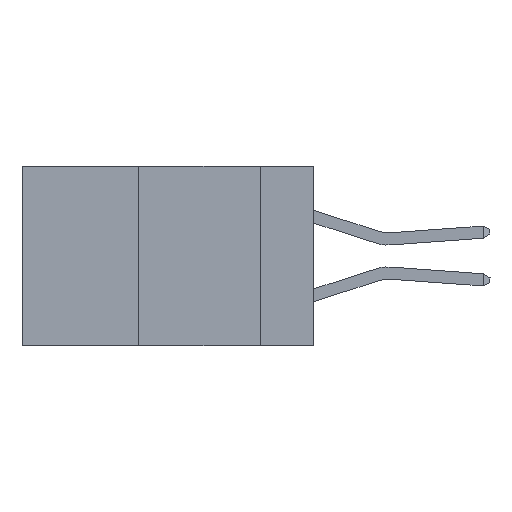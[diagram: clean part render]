
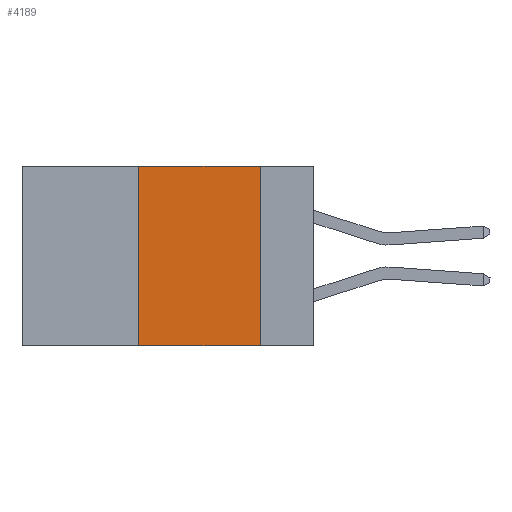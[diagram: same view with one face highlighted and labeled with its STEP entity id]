
A CAD part, left-side view. The second image highlights one B-rep face of the part: STEP entity #4189.
In plain terms, the highlighted planar face has unit normal (-1, 0, 0).
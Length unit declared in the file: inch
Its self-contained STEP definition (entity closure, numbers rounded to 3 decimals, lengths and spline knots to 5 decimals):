
#8 = ORIENTED_EDGE ( 'NONE', *, *, #7872, .F. ) ;
#9 = VECTOR ( 'NONE', #5350, 39.37008 ) ;
#285 = LINE ( 'NONE', #4458, #9 ) ;
#1964 = DIRECTION ( 'NONE',  ( 0., 0., -1. ) ) ;
#1965 = DIRECTION ( 'NONE',  ( 1., 0., 0. ) ) ;
#2003 = CARTESIAN_POINT ( 'NONE',  ( 0., 0.6, 0. ) ) ;
#2019 = DIRECTION ( 'NONE',  ( 0., -1., 0. ) ) ;
#2075 = PLANE ( 'NONE',  #4719 ) ;
#2147 = CARTESIAN_POINT ( 'NONE',  ( 0., 0.11, -0.37 ) ) ;
#2339 = VERTEX_POINT ( 'NONE', #8652 ) ;
#2706 = VECTOR ( 'NONE', #9809, 39.37008 ) ;
#4037 = EDGE_CURVE ( 'NONE', #6255, #4194, #9023, .T. ) ;
#4189 = ADVANCED_FACE ( 'NONE', ( #9587 ), #2075, .F. ) ;
#4194 = VERTEX_POINT ( 'NONE', #2147 ) ;
#4449 = VECTOR ( 'NONE', #2019, 39.37008 ) ;
#4458 = CARTESIAN_POINT ( 'NONE',  ( 0., 0.6, 0. ) ) ;
#4597 = CARTESIAN_POINT ( 'NONE',  ( 0., 0.6, -0.37 ) ) ;
#4719 = AXIS2_PLACEMENT_3D ( 'NONE', #2003, #1965, #1964 ) ;
#4953 = CARTESIAN_POINT ( 'NONE',  ( 0., 0.36, 0. ) ) ;
#5127 = VECTOR ( 'NONE', #8448, 39.37008 ) ;
#5350 = DIRECTION ( 'NONE',  ( 0., -1., 0. ) ) ;
#5508 = ORIENTED_EDGE ( 'NONE', *, *, #6180, .F. ) ;
#6139 = LINE ( 'NONE', #6265, #5127 ) ;
#6180 = EDGE_CURVE ( 'NONE', #6653, #6255, #285, .T. ) ;
#6193 = CARTESIAN_POINT ( 'NONE',  ( 0., 0.11, 0. ) ) ;
#6255 = VERTEX_POINT ( 'NONE', #6193 ) ;
#6265 = CARTESIAN_POINT ( 'NONE',  ( 0., 0.36, 0. ) ) ;
#6653 = VERTEX_POINT ( 'NONE', #4953 ) ;
#7194 = EDGE_CURVE ( 'NONE', #2339, #4194, #8516, .T. ) ;
#7687 = ORIENTED_EDGE ( 'NONE', *, *, #7194, .T. ) ;
#7872 = EDGE_CURVE ( 'NONE', #2339, #6653, #6139, .T. ) ;
#8157 = EDGE_LOOP ( 'NONE', ( #9813, #5508, #8, #7687 ) ) ;
#8448 = DIRECTION ( 'NONE',  ( 0., 0., 1. ) ) ;
#8516 = LINE ( 'NONE', #4597, #4449 ) ;
#8652 = CARTESIAN_POINT ( 'NONE',  ( 0., 0.36, -0.37 ) ) ;
#9023 = LINE ( 'NONE', #9852, #2706 ) ;
#9587 = FACE_OUTER_BOUND ( 'NONE', #8157, .T. ) ;
#9809 = DIRECTION ( 'NONE',  ( 0., 0., -1. ) ) ;
#9813 = ORIENTED_EDGE ( 'NONE', *, *, #4037, .F. ) ;
#9852 = CARTESIAN_POINT ( 'NONE',  ( 0., 0.11, 0. ) ) ;
